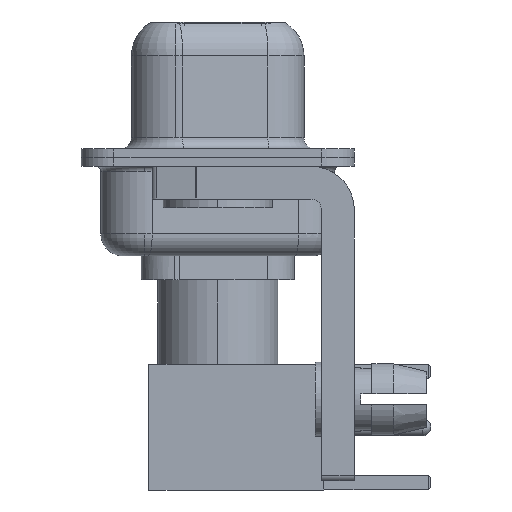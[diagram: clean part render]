
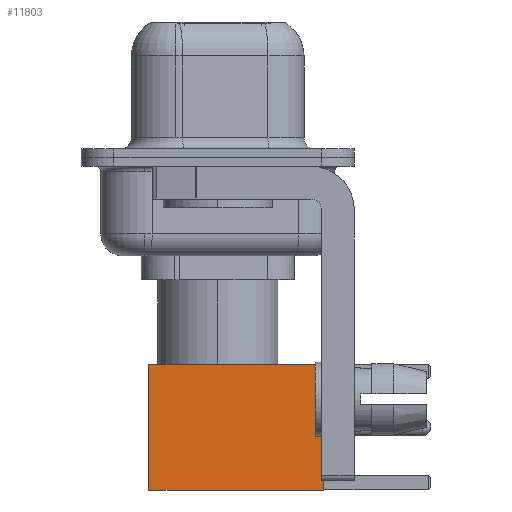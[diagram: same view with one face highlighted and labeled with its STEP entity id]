
A CAD part, left-side view. The second image highlights one B-rep face of the part: STEP entity #11803.
In plain terms, the highlighted face is planar.
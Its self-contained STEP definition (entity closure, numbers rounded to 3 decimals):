
#1742 = CARTESIAN_POINT ( 'NONE',  ( 0., 2.875, 8. ) ) ;
#2007 = DIRECTION ( 'NONE',  ( -1., 0., 0. ) ) ;
#2041 = PLANE ( 'NONE',  #18992 ) ;
#2179 = VERTEX_POINT ( 'NONE', #5810 ) ;
#2230 = LINE ( 'NONE', #14737, #2780 ) ;
#2457 = LINE ( 'NONE', #3917, #5980 ) ;
#2780 = VECTOR ( 'NONE', #2007, 1000. ) ;
#3722 = FACE_OUTER_BOUND ( 'NONE', #10232, .T. ) ;
#3798 = ORIENTED_EDGE ( 'NONE', *, *, #8078, .F. ) ;
#3917 = CARTESIAN_POINT ( 'NONE',  ( -2.875, 2.875, 0. ) ) ;
#4913 = DIRECTION ( 'NONE',  ( -1., 0., 0. ) ) ;
#5800 = EDGE_CURVE ( 'NONE', #13847, #16165, #2230, .T. ) ;
#5810 = CARTESIAN_POINT ( 'NONE',  ( 2.875, 2.875, 8. ) ) ;
#5971 = DIRECTION ( 'NONE',  ( 0., 0., -1. ) ) ;
#5980 = VECTOR ( 'NONE', #15087, 1000. ) ;
#6155 = CARTESIAN_POINT ( 'NONE',  ( 2.875, 2.875, 0. ) ) ;
#6769 = EDGE_CURVE ( 'NONE', #17684, #16165, #2457, .T. ) ;
#6879 = CARTESIAN_POINT ( 'NONE',  ( 2.875, 2.875, 0. ) ) ;
#7857 = EDGE_CURVE ( 'NONE', #2179, #13847, #12284, .T. ) ;
#7963 = LINE ( 'NONE', #1742, #9170 ) ;
#8078 = EDGE_CURVE ( 'NONE', #2179, #17684, #7963, .T. ) ;
#9170 = VECTOR ( 'NONE', #4913, 1000. ) ;
#10232 = EDGE_LOOP ( 'NONE', ( #13256, #18622, #16128, #3798 ) ) ;
#10390 = CARTESIAN_POINT ( 'NONE',  ( 2.875, 2.875, 0. ) ) ;
#11803 = ADVANCED_FACE ( 'NONE', ( #3722 ), #2041, .T. ) ;
#12284 = LINE ( 'NONE', #10390, #19578 ) ;
#12682 = CARTESIAN_POINT ( 'NONE',  ( -2.875, 2.875, 8. ) ) ;
#13256 = ORIENTED_EDGE ( 'NONE', *, *, #7857, .T. ) ;
#13452 = CARTESIAN_POINT ( 'NONE',  ( -2.875, 2.875, 0. ) ) ;
#13847 = VERTEX_POINT ( 'NONE', #6155 ) ;
#14737 = CARTESIAN_POINT ( 'NONE',  ( 0., 2.875, 0. ) ) ;
#15087 = DIRECTION ( 'NONE',  ( 0., 0., -1. ) ) ;
#16128 = ORIENTED_EDGE ( 'NONE', *, *, #6769, .F. ) ;
#16165 = VERTEX_POINT ( 'NONE', #13452 ) ;
#17684 = VERTEX_POINT ( 'NONE', #12682 ) ;
#18622 = ORIENTED_EDGE ( 'NONE', *, *, #5800, .T. ) ;
#18992 = AXIS2_PLACEMENT_3D ( 'NONE', #6879, #19737, #19522 ) ;
#19522 = DIRECTION ( 'NONE',  ( 0., 0., 1. ) ) ;
#19578 = VECTOR ( 'NONE', #5971, 1000. ) ;
#19737 = DIRECTION ( 'NONE',  ( 0., 1., 0. ) ) ;
